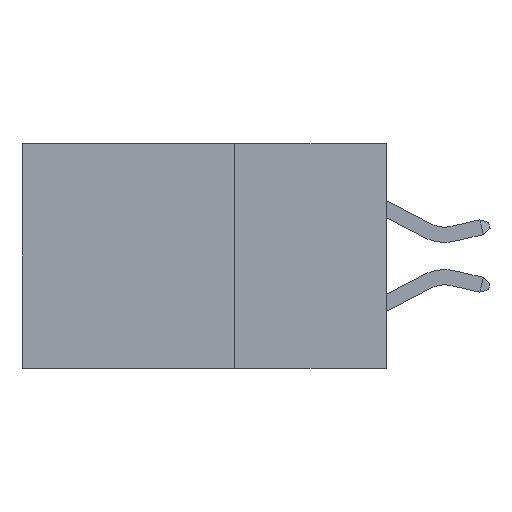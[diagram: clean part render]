
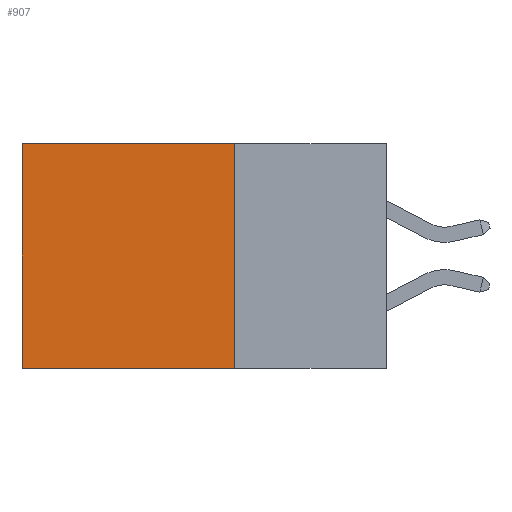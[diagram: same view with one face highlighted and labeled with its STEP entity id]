
A CAD part, left-side view. The second image highlights one B-rep face of the part: STEP entity #907.
In plain terms, the highlighted planar face has unit normal (-1, 0, 0).
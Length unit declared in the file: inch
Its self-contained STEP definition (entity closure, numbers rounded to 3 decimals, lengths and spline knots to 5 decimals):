
#25 = VECTOR ( 'NONE', #11643, 39.37008 ) ;
#35 = VECTOR ( 'NONE', #7555, 39.37008 ) ;
#284 = EDGE_CURVE ( 'NONE', #430, #4675, #2689, .T. ) ;
#416 = EDGE_CURVE ( 'NONE', #430, #1755, #1997, .T. ) ;
#430 = VERTEX_POINT ( 'NONE', #11422 ) ;
#433 = CARTESIAN_POINT ( 'NONE',  ( 0.298, 0.25, -0.37 ) ) ;
#907 = ADVANCED_FACE ( 'NONE', ( #4469 ), #1644, .F. ) ;
#1644 = PLANE ( 'NONE',  #6046 ) ;
#1720 = VECTOR ( 'NONE', #11749, 39.37008 ) ;
#1755 = VERTEX_POINT ( 'NONE', #11543 ) ;
#1782 = ORIENTED_EDGE ( 'NONE', *, *, #6005, .F. ) ;
#1997 = LINE ( 'NONE', #8738, #1720 ) ;
#2204 = ORIENTED_EDGE ( 'NONE', *, *, #416, .T. ) ;
#2689 = LINE ( 'NONE', #6608, #25 ) ;
#3033 = EDGE_CURVE ( 'NONE', #1755, #10852, #5516, .T. ) ;
#3270 = CARTESIAN_POINT ( 'NONE',  ( 0.298, 0.25, -0.37 ) ) ;
#4469 = FACE_OUTER_BOUND ( 'NONE', #8606, .T. ) ;
#4637 = ORIENTED_EDGE ( 'NONE', *, *, #284, .F. ) ;
#4675 = VERTEX_POINT ( 'NONE', #433 ) ;
#5516 = LINE ( 'NONE', #9523, #7666 ) ;
#5580 = ORIENTED_EDGE ( 'NONE', *, *, #3033, .T. ) ;
#6005 = EDGE_CURVE ( 'NONE', #4675, #10852, #7525, .T. ) ;
#6046 = AXIS2_PLACEMENT_3D ( 'NONE', #9726, #8081, #9522 ) ;
#6608 = CARTESIAN_POINT ( 'NONE',  ( 0.298, 0.25, 0. ) ) ;
#7525 = LINE ( 'NONE', #3270, #35 ) ;
#7555 = DIRECTION ( 'NONE',  ( 0., 1., 0. ) ) ;
#7666 = VECTOR ( 'NONE', #9525, 39.37008 ) ;
#8081 = DIRECTION ( 'NONE',  ( 1., 0., 0. ) ) ;
#8606 = EDGE_LOOP ( 'NONE', ( #5580, #1782, #4637, #2204 ) ) ;
#8738 = CARTESIAN_POINT ( 'NONE',  ( 0.298, 0.25, 0. ) ) ;
#9522 = DIRECTION ( 'NONE',  ( 0., 0., -1. ) ) ;
#9523 = CARTESIAN_POINT ( 'NONE',  ( 0.298, 0.6, 0. ) ) ;
#9525 = DIRECTION ( 'NONE',  ( 0., 0., -1. ) ) ;
#9726 = CARTESIAN_POINT ( 'NONE',  ( 0.298, 0.25, 0. ) ) ;
#10852 = VERTEX_POINT ( 'NONE', #11799 ) ;
#11422 = CARTESIAN_POINT ( 'NONE',  ( 0.298, 0.25, 0. ) ) ;
#11543 = CARTESIAN_POINT ( 'NONE',  ( 0.298, 0.6, 0. ) ) ;
#11643 = DIRECTION ( 'NONE',  ( 0., 0., -1. ) ) ;
#11749 = DIRECTION ( 'NONE',  ( 0., 1., 0. ) ) ;
#11799 = CARTESIAN_POINT ( 'NONE',  ( 0.298, 0.6, -0.37 ) ) ;
